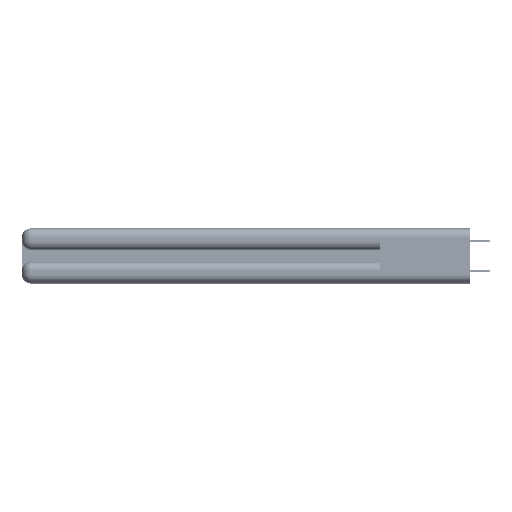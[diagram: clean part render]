
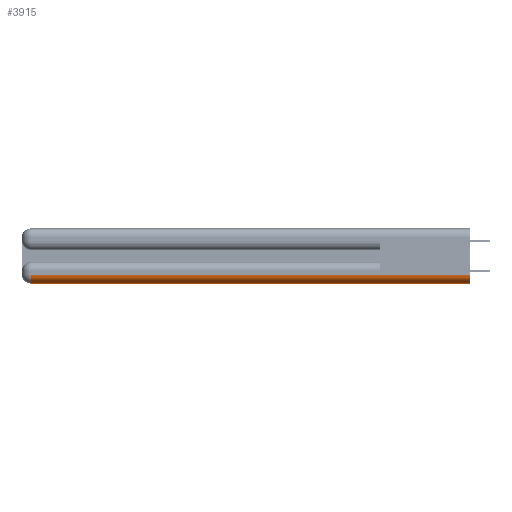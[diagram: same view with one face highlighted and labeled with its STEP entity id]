
A CAD part, left-side view. The second image highlights one B-rep face of the part: STEP entity #3915.
In plain terms, the highlighted cylindrical face has radius 1.524 mm (diameter 3.048 mm), a partial arc.
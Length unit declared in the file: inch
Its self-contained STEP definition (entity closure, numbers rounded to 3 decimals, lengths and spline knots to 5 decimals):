
#2468 = CARTESIAN_POINT ( 'NONE',  ( 0.06, 0., 0.06 ) ) ;
#3138 = VERTEX_POINT ( 'NONE', #40423 ) ;
#3915 = ADVANCED_FACE ( 'NONE', ( #56043 ), #34882, .T. ) ;
#6725 = EDGE_CURVE ( 'NONE', #30258, #3138, #17275, .T. ) ;
#7879 = CIRCLE ( 'NONE', #39810, 0.06 ) ;
#10220 = VECTOR ( 'NONE', #39394, 39.37008 ) ;
#12598 = CARTESIAN_POINT ( 'NONE',  ( 0.06, 2.94, 0.06 ) ) ;
#13711 = CARTESIAN_POINT ( 'NONE',  ( 0., 0., 0.06 ) ) ;
#16450 = DIRECTION ( 'NONE',  ( 0., 1., 0. ) ) ;
#16610 = VERTEX_POINT ( 'NONE', #13711 ) ;
#17275 = LINE ( 'NONE', #21012, #49075 ) ;
#18771 = LINE ( 'NONE', #35651, #10220 ) ;
#19914 = DIRECTION ( 'NONE',  ( 0., -1., 0. ) ) ;
#21012 = CARTESIAN_POINT ( 'NONE',  ( 0.06, 3., 0. ) ) ;
#22150 = ORIENTED_EDGE ( 'NONE', *, *, #47084, .F. ) ;
#24770 = DIRECTION ( 'NONE',  ( 0., 0., 1. ) ) ;
#25601 = ORIENTED_EDGE ( 'NONE', *, *, #6725, .F. ) ;
#28028 = ORIENTED_EDGE ( 'NONE', *, *, #53824, .F. ) ;
#30258 = VERTEX_POINT ( 'NONE', #43277 ) ;
#30587 = DIRECTION ( 'NONE',  ( 0., 1., 0. ) ) ;
#32088 = CIRCLE ( 'NONE', #39428, 0.06 ) ;
#34596 = CARTESIAN_POINT ( 'NONE',  ( 0.06, 0., 0.06 ) ) ;
#34882 = CYLINDRICAL_SURFACE ( 'NONE', #47193, 0.06 ) ;
#35651 = CARTESIAN_POINT ( 'NONE',  ( 0., 0., 0.06 ) ) ;
#36736 = EDGE_CURVE ( 'NONE', #16610, #30258, #32088, .T. ) ;
#39394 = DIRECTION ( 'NONE',  ( 0., -1., 0. ) ) ;
#39428 = AXIS2_PLACEMENT_3D ( 'NONE', #2468, #19914, #24770 ) ;
#39810 = AXIS2_PLACEMENT_3D ( 'NONE', #12598, #30587, #51491 ) ;
#40423 = CARTESIAN_POINT ( 'NONE',  ( 0.06, 2.94, 0. ) ) ;
#40964 = ORIENTED_EDGE ( 'NONE', *, *, #36736, .F. ) ;
#43277 = CARTESIAN_POINT ( 'NONE',  ( 0.06, 0., 0. ) ) ;
#43439 = VERTEX_POINT ( 'NONE', #51486 ) ;
#44639 = EDGE_LOOP ( 'NONE', ( #40964, #22150, #28028, #25601 ) ) ;
#47084 = EDGE_CURVE ( 'NONE', #43439, #16610, #18771, .T. ) ;
#47193 = AXIS2_PLACEMENT_3D ( 'NONE', #34596, #55471, #51749 ) ;
#49075 = VECTOR ( 'NONE', #16450, 39.37008 ) ;
#51486 = CARTESIAN_POINT ( 'NONE',  ( 0., 2.94, 0.06 ) ) ;
#51491 = DIRECTION ( 'NONE',  ( 0., 0., 1. ) ) ;
#51749 = DIRECTION ( 'NONE',  ( 0., 0., 1. ) ) ;
#53824 = EDGE_CURVE ( 'NONE', #3138, #43439, #7879, .T. ) ;
#55471 = DIRECTION ( 'NONE',  ( 0., 1., 0. ) ) ;
#56043 = FACE_OUTER_BOUND ( 'NONE', #44639, .T. ) ;
